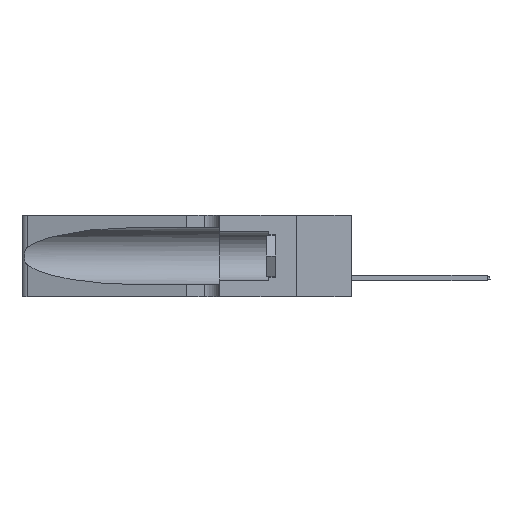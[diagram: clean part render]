
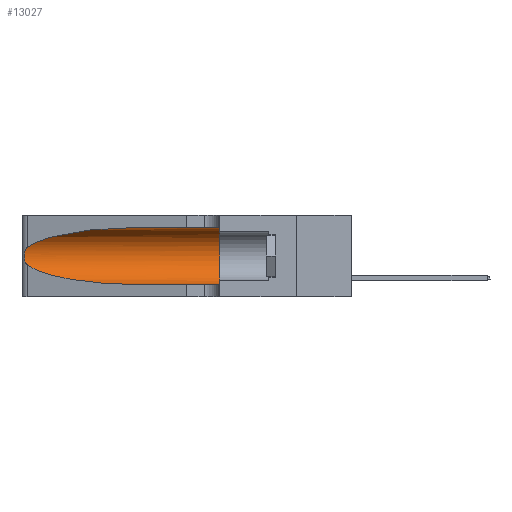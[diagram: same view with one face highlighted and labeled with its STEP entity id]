
A CAD part, left-side view. The second image highlights one B-rep face of the part: STEP entity #13027.
In plain terms, the highlighted cylindrical face has radius 3.308 mm (diameter 6.617 mm), a partial arc.
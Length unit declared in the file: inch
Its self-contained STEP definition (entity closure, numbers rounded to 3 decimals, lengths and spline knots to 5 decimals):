
#356 = VERTEX_POINT ( 'NONE', #1956 ) ;
#1935 = AXIS2_PLACEMENT_3D ( 'NONE', #2850, #13918, #6779 ) ;
#1956 = CARTESIAN_POINT ( 'NONE',  ( 0.1305, 0.35, 0.05475 ) ) ;
#2024 = ORIENTED_EDGE ( 'NONE', *, *, #9076, .T. ) ;
#2071 = AXIS2_PLACEMENT_3D ( 'NONE', #18023, #22766, #9176 ) ;
#2713 = FACE_OUTER_BOUND ( 'NONE', #17168, .T. ) ;
#2849 = CIRCLE ( 'NONE', #2071, 0.13025 ) ;
#2850 = CARTESIAN_POINT ( 'NONE',  ( 0.1305, 1.61858, 0.185 ) ) ;
#3029 = CARTESIAN_POINT ( 'NONE',  ( 0.25856, 1.23593, 0.16098 ) ) ;
#3065 = ORIENTED_EDGE ( 'NONE', *, *, #9248, .F. ) ;
#3747 = VERTEX_POINT ( 'NONE', #8476 ) ;
#3788 = ORIENTED_EDGE ( 'NONE', *, *, #5144, .T. ) ;
#4829 = CARTESIAN_POINT ( 'NONE',  ( 0.25639, 1.23186, 0.15144 ) ) ;
#4857 = VERTEX_POINT ( 'NONE', #20526 ) ;
#5129 = CARTESIAN_POINT ( 'NONE',  ( 0.18966, 0.96281, 0.05475 ) ) ;
#5144 = EDGE_CURVE ( 'NONE', #4857, #21310, #18360, .T. ) ;
#5216 = ORIENTED_EDGE ( 'NONE', *, *, #8873, .F. ) ;
#6248 = CARTESIAN_POINT ( 'NONE',  ( 0.25555, 1.22994, 0.2215 ) ) ;
#6325 = CARTESIAN_POINT ( 'NONE',  ( 0.26075, 1.23896, 0.178 ) ) ;
#6397 = CARTESIAN_POINT ( 'NONE',  ( 0.26018, 1.23835, 0.19895 ) ) ;
#6500 = CARTESIAN_POINT ( 'NONE',  ( 0.1305, 1.61858, 0.05475 ) ) ;
#6615 = CARTESIAN_POINT ( 'NONE',  ( 0.1305, 0.72297, 0.31525 ) ) ;
#6779 = DIRECTION ( 'NONE',  ( 0., 0., -1. ) ) ;
#6935 = CARTESIAN_POINT ( 'NONE',  ( 0.25487, 1.22718, 0.14631 ) ) ;
#7714 = DIRECTION ( 'NONE',  ( 0., -1., 0. ) ) ;
#8476 = CARTESIAN_POINT ( 'NONE',  ( 0.1305, 0.35, 0.31525 ) ) ;
#8529 = CARTESIAN_POINT ( 'NONE',  ( 0.18966, 0.96281, 0.31525 ) ) ;
#8873 = EDGE_CURVE ( 'NONE', #3747, #356, #2849, .T. ) ;
#9076 = EDGE_CURVE ( 'NONE', #14585, #16315, #9331, .T. ) ;
#9176 = DIRECTION ( 'NONE',  ( 0., 0., 1. ) ) ;
#9248 = EDGE_CURVE ( 'NONE', #14585, #3747, #19659, .T. ) ;
#9331 =( BOUNDED_CURVE ( )  B_SPLINE_CURVE ( 3, ( #6615, #8529, #22926, #13696 ),
 .UNSPECIFIED., .F., .F. ) 
 B_SPLINE_CURVE_WITH_KNOTS ( ( 4, 4 ),
 ( 1.5708, 2.84003 ),
 .UNSPECIFIED. ) 
 CURVE ( )  GEOMETRIC_REPRESENTATION_ITEM ( )  RATIONAL_B_SPLINE_CURVE ( ( 1., 0.87, 0.87, 1. ) ) 
 REPRESENTATION_ITEM ( '' )  );
#9678 = EDGE_CURVE ( 'NONE', #21310, #356, #17942, .T. ) ;
#9691 = CARTESIAN_POINT ( 'NONE',  ( 0.1305, 1.61858, 0.31525 ) ) ;
#10573 = CARTESIAN_POINT ( 'NONE',  ( 0.1305, 0.72297, 0.05475 ) ) ;
#11074 = ORIENTED_EDGE ( 'NONE', *, *, #17423, .T. ) ;
#12169 = DIRECTION ( 'NONE',  ( 0., -1., 0. ) ) ;
#13027 = ADVANCED_FACE ( 'NONE', ( #2713 ), #21749, .F. ) ;
#13410 = CARTESIAN_POINT ( 'NONE',  ( 0.25487, 1.22718, 0.22369 ) ) ;
#13632 = CARTESIAN_POINT ( 'NONE',  ( 0.25854, 1.2359, 0.20912 ) ) ;
#13696 = CARTESIAN_POINT ( 'NONE',  ( 0.25487, 1.22718, 0.22369 ) ) ;
#13781 = CARTESIAN_POINT ( 'NONE',  ( 0.26075, 1.23896, 0.19203 ) ) ;
#13918 = DIRECTION ( 'NONE',  ( 0., -1., 0. ) ) ;
#14033 = CARTESIAN_POINT ( 'NONE',  ( 0.1305, 0.72297, 0.31525 ) ) ;
#14207 = B_SPLINE_CURVE_WITH_KNOTS ( 'NONE', 3,
 ( #13410, #6248, #18735, #22558, #13632, #6397, #13781, #6325, #20677, #3029, #15582, #4829, #22483, #17209 ),
 .UNSPECIFIED., .F., .F.,
 ( 4, 2, 2, 2, 2, 2, 4 ),
 ( 0., 0.00027, 0.00053, 0.00107, 0.0016, 0.00187, 0.00214 ),
 .UNSPECIFIED. ) ;
#14585 = VERTEX_POINT ( 'NONE', #14033 ) ;
#14916 = VECTOR ( 'NONE', #7714, 39.37008 ) ;
#15582 = CARTESIAN_POINT ( 'NONE',  ( 0.25789, 1.23486, 0.15765 ) ) ;
#16315 = VERTEX_POINT ( 'NONE', #21206 ) ;
#17168 = EDGE_LOOP ( 'NONE', ( #2024, #11074, #3788, #21152, #5216, #3065 ) ) ;
#17209 = CARTESIAN_POINT ( 'NONE',  ( 0.25487, 1.22718, 0.14631 ) ) ;
#17423 = EDGE_CURVE ( 'NONE', #16315, #4857, #14207, .T. ) ;
#17942 = LINE ( 'NONE', #6500, #20208 ) ;
#18023 = CARTESIAN_POINT ( 'NONE',  ( 0.1305, 0.35, 0.185 ) ) ;
#18360 =( BOUNDED_CURVE ( )  B_SPLINE_CURVE ( 3, ( #6935, #23014, #5129, #10573 ),
 .UNSPECIFIED., .F., .F. ) 
 B_SPLINE_CURVE_WITH_KNOTS ( ( 4, 4 ),
 ( 3.44316, 4.71239 ),
 .UNSPECIFIED. ) 
 CURVE ( )  GEOMETRIC_REPRESENTATION_ITEM ( )  RATIONAL_B_SPLINE_CURVE ( ( 1., 0.87, 0.87, 1. ) ) 
 REPRESENTATION_ITEM ( '' )  );
#18735 = CARTESIAN_POINT ( 'NONE',  ( 0.25639, 1.23184, 0.21858 ) ) ;
#19659 = LINE ( 'NONE', #9691, #14916 ) ;
#19803 = CARTESIAN_POINT ( 'NONE',  ( 0.1305, 0.72297, 0.05475 ) ) ;
#20208 = VECTOR ( 'NONE', #12169, 39.37008 ) ;
#20526 = CARTESIAN_POINT ( 'NONE',  ( 0.25487, 1.22718, 0.14631 ) ) ;
#20677 = CARTESIAN_POINT ( 'NONE',  ( 0.26017, 1.23833, 0.17102 ) ) ;
#21152 = ORIENTED_EDGE ( 'NONE', *, *, #9678, .T. ) ;
#21206 = CARTESIAN_POINT ( 'NONE',  ( 0.25487, 1.22718, 0.22369 ) ) ;
#21310 = VERTEX_POINT ( 'NONE', #19803 ) ;
#21749 = CYLINDRICAL_SURFACE ( 'NONE', #1935, 0.13025 ) ;
#22483 = CARTESIAN_POINT ( 'NONE',  ( 0.25555, 1.22993, 0.14849 ) ) ;
#22558 = CARTESIAN_POINT ( 'NONE',  ( 0.25787, 1.23484, 0.2124 ) ) ;
#22766 = DIRECTION ( 'NONE',  ( 0., 1., 0. ) ) ;
#22926 = CARTESIAN_POINT ( 'NONE',  ( 0.2373, 1.15595, 0.28018 ) ) ;
#23014 = CARTESIAN_POINT ( 'NONE',  ( 0.2373, 1.15595, 0.08982 ) ) ;
